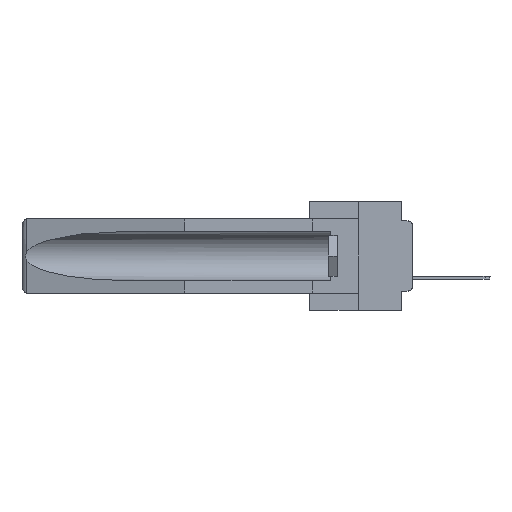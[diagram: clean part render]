
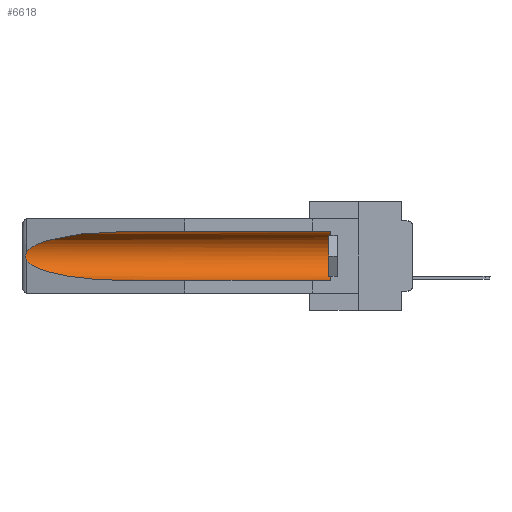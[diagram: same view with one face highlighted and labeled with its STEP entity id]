
A CAD part, left-side view. The second image highlights one B-rep face of the part: STEP entity #6618.
In plain terms, the highlighted cylindrical face has radius 2.857 mm (diameter 5.715 mm), a partial arc.
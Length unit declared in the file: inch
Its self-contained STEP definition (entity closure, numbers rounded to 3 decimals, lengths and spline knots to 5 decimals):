
#337 = LINE ( 'NONE', #10371, #16967 ) ;
#467 = DIRECTION ( 'NONE',  ( 0., 1., 0. ) ) ;
#2021 = CARTESIAN_POINT ( 'NONE',  ( 0.26537, 1.52718, -0.14972 ) ) ;
#2363 = EDGE_CURVE ( 'NONE', #5952, #11259, #19217, .T. ) ;
#2625 = CARTESIAN_POINT ( 'NONE',  ( 0.26537, 1.52718, -0.19328 ) ) ;
#3997 = CARTESIAN_POINT ( 'NONE',  ( 0.2673, 1.53269, -0.17917 ) ) ;
#5952 = VERTEX_POINT ( 'NONE', #23197 ) ;
#6063 = VERTEX_POINT ( 'NONE', #8572 ) ;
#6410 = ORIENTED_EDGE ( 'NONE', *, *, #14613, .T. ) ;
#6471 = CARTESIAN_POINT ( 'NONE',  ( 0.26597, 1.52961, -0.15275 ) ) ;
#6618 = ADVANCED_FACE ( 'NONE', ( #21672 ), #8842, .F. ) ;
#7800 = DIRECTION ( 'NONE',  ( 0., 0., 1. ) ) ;
#7955 = CARTESIAN_POINT ( 'NONE',  ( 0.25451, 1.48313, -0.24835 ) ) ;
#8482 = CARTESIAN_POINT ( 'NONE',  ( 0.25451, 1.48313, -0.09465 ) ) ;
#8572 = CARTESIAN_POINT ( 'NONE',  ( 0.155, 1.07973, -0.059 ) ) ;
#8842 = CYLINDRICAL_SURFACE ( 'NONE', #24784, 0.1125 ) ;
#9248 = CARTESIAN_POINT ( 'NONE',  ( 0.155, 1.07973, -0.059 ) ) ;
#9418 = CARTESIAN_POINT ( 'NONE',  ( 0.2675, 1.53308, -0.16763 ) ) ;
#9503 = CARTESIAN_POINT ( 'NONE',  ( 0.155, 1.07973, -0.284 ) ) ;
#10046 = CARTESIAN_POINT ( 'NONE',  ( 0.155, 0.126, -0.059 ) ) ;
#10255 = DIRECTION ( 'NONE',  ( 0., -1., 0. ) ) ;
#10371 = CARTESIAN_POINT ( 'NONE',  ( 0.155, -0.30754, -0.284 ) ) ;
#10776 =( BOUNDED_CURVE ( )  B_SPLINE_CURVE ( 3, ( #23387, #7955, #17984, #23069 ),
 .UNSPECIFIED., .F., .T. ) 
 B_SPLINE_CURVE_WITH_KNOTS ( ( 4, 4 ),
 ( 0.1948, 1.5708 ),
 .UNSPECIFIED. ) 
 CURVE ( )  GEOMETRIC_REPRESENTATION_ITEM ( )  RATIONAL_B_SPLINE_CURVE ( ( 1., 0.848, 0.848, 1. ) ) 
 REPRESENTATION_ITEM ( '' )  );
#10988 = CARTESIAN_POINT ( 'NONE',  ( 0.155, -0.30754, -0.059 ) ) ;
#11259 = VERTEX_POINT ( 'NONE', #2625 ) ;
#11834 = ORIENTED_EDGE ( 'NONE', *, *, #16778, .T. ) ;
#11880 = CARTESIAN_POINT ( 'NONE',  ( 0.26655, 1.53094, -0.18657 ) ) ;
#13167 = VECTOR ( 'NONE', #467, 39.37008 ) ;
#13364 = EDGE_CURVE ( 'NONE', #11259, #29285, #10776, .T. ) ;
#13599 = VERTEX_POINT ( 'NONE', #10046 ) ;
#14186 = CARTESIAN_POINT ( 'NONE',  ( 0.26654, 1.53092, -0.15636 ) ) ;
#14607 = CIRCLE ( 'NONE', #22495, 0.1125 ) ;
#14613 = EDGE_CURVE ( 'NONE', #26097, #13599, #14607, .T. ) ;
#15767 = LINE ( 'NONE', #10988, #13167 ) ;
#16142 = EDGE_CURVE ( 'NONE', #6063, #5952, #18584, .T. ) ;
#16498 = CARTESIAN_POINT ( 'NONE',  ( 0.2675, 1.53308, -0.17534 ) ) ;
#16778 = EDGE_CURVE ( 'NONE', #13599, #6063, #15767, .T. ) ;
#16831 = CARTESIAN_POINT ( 'NONE',  ( 0.26597, 1.5296, -0.19026 ) ) ;
#16967 = VECTOR ( 'NONE', #27976, 39.37008 ) ;
#17216 = DIRECTION ( 'NONE',  ( 0., 0., 1. ) ) ;
#17984 = CARTESIAN_POINT ( 'NONE',  ( 0.21114, 1.30732, -0.284 ) ) ;
#18396 = ORIENTED_EDGE ( 'NONE', *, *, #13364, .T. ) ;
#18573 = CARTESIAN_POINT ( 'NONE',  ( 0.155, -0.30754, -0.1715 ) ) ;
#18584 =( BOUNDED_CURVE ( )  B_SPLINE_CURVE ( 3, ( #9248, #24523, #8482, #31987 ),
 .UNSPECIFIED., .F., .F. ) 
 B_SPLINE_CURVE_WITH_KNOTS ( ( 4, 4 ),
 ( 4.71239, 6.08839 ),
 .UNSPECIFIED. ) 
 CURVE ( )  GEOMETRIC_REPRESENTATION_ITEM ( )  RATIONAL_B_SPLINE_CURVE ( ( 1., 0.848, 0.848, 1. ) ) 
 REPRESENTATION_ITEM ( '' )  );
#19217 = B_SPLINE_CURVE_WITH_KNOTS ( 'NONE', 3,
 ( #2021, #6471, #14186, #24528, #9418, #16498, #3997, #11880, #16831, #19450 ),
 .UNSPECIFIED., .F., .F.,
 ( 4, 2, 2, 2, 4 ),
 ( 0., 0.00029, 0.00058, 0.00087, 0.00117 ),
 .UNSPECIFIED. ) ;
#19450 = CARTESIAN_POINT ( 'NONE',  ( 0.26537, 1.52718, -0.19328 ) ) ;
#21672 = FACE_OUTER_BOUND ( 'NONE', #27219, .T. ) ;
#22495 = AXIS2_PLACEMENT_3D ( 'NONE', #30505, #10255, #7800 ) ;
#23069 = CARTESIAN_POINT ( 'NONE',  ( 0.155, 1.07973, -0.284 ) ) ;
#23146 = ORIENTED_EDGE ( 'NONE', *, *, #16142, .T. ) ;
#23197 = CARTESIAN_POINT ( 'NONE',  ( 0.26537, 1.52718, -0.14972 ) ) ;
#23387 = CARTESIAN_POINT ( 'NONE',  ( 0.26537, 1.52718, -0.19328 ) ) ;
#24523 = CARTESIAN_POINT ( 'NONE',  ( 0.21114, 1.30732, -0.059 ) ) ;
#24528 = CARTESIAN_POINT ( 'NONE',  ( 0.2673, 1.5327, -0.16383 ) ) ;
#24784 = AXIS2_PLACEMENT_3D ( 'NONE', #18573, #28607, #17216 ) ;
#24962 = EDGE_CURVE ( 'NONE', #26097, #29285, #337, .T. ) ;
#25752 = ORIENTED_EDGE ( 'NONE', *, *, #2363, .T. ) ;
#26097 = VERTEX_POINT ( 'NONE', #32462 ) ;
#27219 = EDGE_LOOP ( 'NONE', ( #23146, #25752, #18396, #31290, #6410, #11834 ) ) ;
#27976 = DIRECTION ( 'NONE',  ( 0., 1., 0. ) ) ;
#28607 = DIRECTION ( 'NONE',  ( 0., 1., 0. ) ) ;
#29285 = VERTEX_POINT ( 'NONE', #9503 ) ;
#30505 = CARTESIAN_POINT ( 'NONE',  ( 0.155, 0.126, -0.1715 ) ) ;
#31290 = ORIENTED_EDGE ( 'NONE', *, *, #24962, .F. ) ;
#31987 = CARTESIAN_POINT ( 'NONE',  ( 0.26537, 1.52718, -0.14972 ) ) ;
#32462 = CARTESIAN_POINT ( 'NONE',  ( 0.155, 0.126, -0.284 ) ) ;
